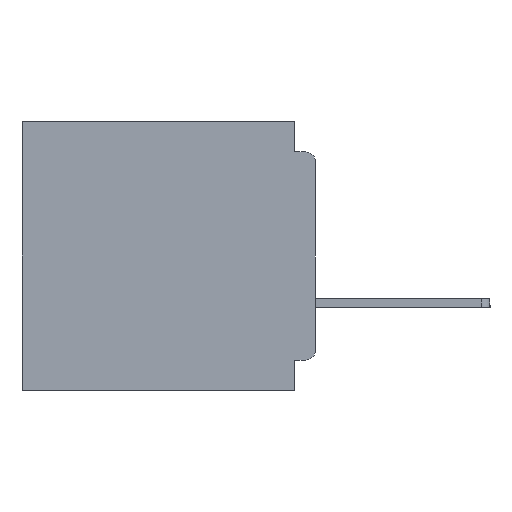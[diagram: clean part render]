
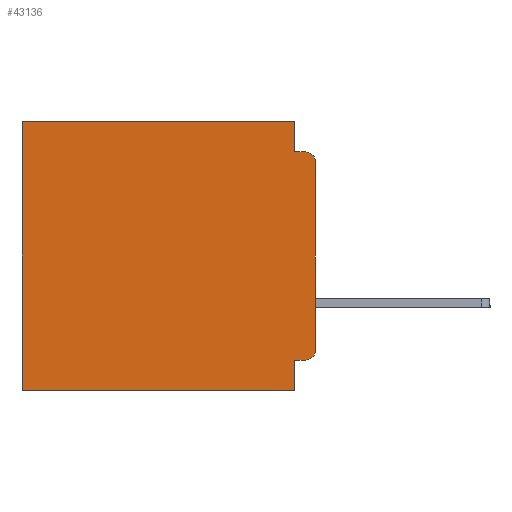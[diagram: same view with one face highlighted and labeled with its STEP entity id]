
A CAD part, left-side view. The second image highlights one B-rep face of the part: STEP entity #43136.
In plain terms, the highlighted planar face has unit normal (-1, 0, 0).
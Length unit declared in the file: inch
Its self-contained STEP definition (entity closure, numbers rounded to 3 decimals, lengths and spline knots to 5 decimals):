
#1209 = VERTEX_POINT ( 'NONE', #57532 ) ;
#2395 = DIRECTION ( 'NONE',  ( 0., 1., 0. ) ) ;
#2938 = VECTOR ( 'NONE', #21959, 39.37008 ) ;
#3122 = ORIENTED_EDGE ( 'NONE', *, *, #51574, .T. ) ;
#3294 = VECTOR ( 'NONE', #12545, 39.37008 ) ;
#3520 = DIRECTION ( 'NONE',  ( 0., 0., -1. ) ) ;
#4760 = DIRECTION ( 'NONE',  ( -1., 0., 0. ) ) ;
#5353 = ORIENTED_EDGE ( 'NONE', *, *, #50218, .F. ) ;
#6563 = CARTESIAN_POINT ( 'NONE',  ( 0.3, 0., 0. ) ) ;
#8400 = CARTESIAN_POINT ( 'NONE',  ( 0.3, 0.437, 0. ) ) ;
#9944 = VERTEX_POINT ( 'NONE', #12247 ) ;
#10645 = CARTESIAN_POINT ( 'NONE',  ( 0.3, 0., -0.4 ) ) ;
#10893 = EDGE_CURVE ( 'NONE', #55177, #16898, #20337, .T. ) ;
#11255 = ORIENTED_EDGE ( 'NONE', *, *, #14312, .F. ) ;
#11325 = DIRECTION ( 'NONE',  ( 0., 1., 0. ) ) ;
#11742 = VERTEX_POINT ( 'NONE', #34514 ) ;
#12247 = CARTESIAN_POINT ( 'NONE',  ( 0.3, 0.031, -0.4 ) ) ;
#12248 = EDGE_CURVE ( 'NONE', #55177, #11742, #18725, .T. ) ;
#12545 = DIRECTION ( 'NONE',  ( 0., 0., -1. ) ) ;
#13112 = ORIENTED_EDGE ( 'NONE', *, *, #36123, .F. ) ;
#14312 = EDGE_CURVE ( 'NONE', #32155, #57522, #51181, .T. ) ;
#15388 = EDGE_CURVE ( 'NONE', #32155, #17351, #39405, .T. ) ;
#15807 = DIRECTION ( 'NONE',  ( 0., 1., 0. ) ) ;
#16235 = ORIENTED_EDGE ( 'NONE', *, *, #10893, .T. ) ;
#16368 = CARTESIAN_POINT ( 'NONE',  ( 0.3, 0., -0.355 ) ) ;
#16898 = VERTEX_POINT ( 'NONE', #42396 ) ;
#16939 = AXIS2_PLACEMENT_3D ( 'NONE', #32776, #4760, #37482 ) ;
#17249 = LINE ( 'NONE', #49866, #3294 ) ;
#17351 = VERTEX_POINT ( 'NONE', #8400 ) ;
#17574 = DIRECTION ( 'NONE',  ( -1., 0., 0. ) ) ;
#18725 = LINE ( 'NONE', #39203, #42150 ) ;
#20140 = EDGE_CURVE ( 'NONE', #1209, #11742, #28100, .T. ) ;
#20337 = CIRCLE ( 'NONE', #16939, 0.015 ) ;
#21219 = ORIENTED_EDGE ( 'NONE', *, *, #20140, .T. ) ;
#21724 = LINE ( 'NONE', #16368, #32735 ) ;
#21959 = DIRECTION ( 'NONE',  ( 0., 0., -1. ) ) ;
#22036 = ORIENTED_EDGE ( 'NONE', *, *, #32426, .F. ) ;
#22217 = LINE ( 'NONE', #31538, #45684 ) ;
#22453 = CARTESIAN_POINT ( 'NONE',  ( 0.3, 0.031, -0.355 ) ) ;
#23153 = LINE ( 'NONE', #50986, #35647 ) ;
#23790 = CARTESIAN_POINT ( 'NONE',  ( 0.3, 0.437, -0.4 ) ) ;
#25708 = ORIENTED_EDGE ( 'NONE', *, *, #12248, .F. ) ;
#27734 = DIRECTION ( 'NONE',  ( 0., -1., 0. ) ) ;
#28100 = CIRCLE ( 'NONE', #52515, 0.015 ) ;
#29387 = DIRECTION ( 'NONE',  ( 0., 0., -1. ) ) ;
#31421 = CARTESIAN_POINT ( 'NONE',  ( 0.3, 0.031, 0. ) ) ;
#31483 = VERTEX_POINT ( 'NONE', #23790 ) ;
#31538 = CARTESIAN_POINT ( 'NONE',  ( 0.3, 0.031, -0.4 ) ) ;
#32155 = VERTEX_POINT ( 'NONE', #43239 ) ;
#32426 = EDGE_CURVE ( 'NONE', #39357, #9944, #22217, .T. ) ;
#32735 = VECTOR ( 'NONE', #2395, 39.37008 ) ;
#32776 = CARTESIAN_POINT ( 'NONE',  ( 0.3, 0.015, -0.06 ) ) ;
#33311 = LINE ( 'NONE', #48467, #56722 ) ;
#34514 = CARTESIAN_POINT ( 'NONE',  ( 0.3, 0., -0.34 ) ) ;
#34724 = AXIS2_PLACEMENT_3D ( 'NONE', #10645, #57430, #29387 ) ;
#35647 = VECTOR ( 'NONE', #27734, 39.37008 ) ;
#35848 = FACE_OUTER_BOUND ( 'NONE', #46391, .T. ) ;
#36123 = EDGE_CURVE ( 'NONE', #57522, #16898, #23153, .T. ) ;
#37439 = CARTESIAN_POINT ( 'NONE',  ( 0.3, 0.031, -0.045 ) ) ;
#37482 = DIRECTION ( 'NONE',  ( 0., 0., -1. ) ) ;
#39203 = CARTESIAN_POINT ( 'NONE',  ( 0.3, 0., -0.4 ) ) ;
#39357 = VERTEX_POINT ( 'NONE', #22453 ) ;
#39405 = LINE ( 'NONE', #6563, #51772 ) ;
#42150 = VECTOR ( 'NONE', #57998, 39.37008 ) ;
#42396 = CARTESIAN_POINT ( 'NONE',  ( 0.3, 0.015, -0.045 ) ) ;
#43136 = ADVANCED_FACE ( 'NONE', ( #35848 ), #43332, .F. ) ;
#43239 = CARTESIAN_POINT ( 'NONE',  ( 0.3, 0.031, 0. ) ) ;
#43332 = PLANE ( 'NONE',  #34724 ) ;
#45026 = ORIENTED_EDGE ( 'NONE', *, *, #15388, .T. ) ;
#45557 = CARTESIAN_POINT ( 'NONE',  ( 0.3, 0.015, -0.34 ) ) ;
#45684 = VECTOR ( 'NONE', #3520, 39.37008 ) ;
#46391 = EDGE_LOOP ( 'NONE', ( #25708, #16235, #13112, #11255, #45026, #3122, #52841, #22036, #5353, #21219 ) ) ;
#48467 = CARTESIAN_POINT ( 'NONE',  ( 0.3, 0., -0.4 ) ) ;
#49866 = CARTESIAN_POINT ( 'NONE',  ( 0.3, 0.437, -0.4 ) ) ;
#50216 = DIRECTION ( 'NONE',  ( 0., 0., -1. ) ) ;
#50218 = EDGE_CURVE ( 'NONE', #1209, #39357, #21724, .T. ) ;
#50986 = CARTESIAN_POINT ( 'NONE',  ( 0.3, 0., -0.045 ) ) ;
#51181 = LINE ( 'NONE', #31421, #2938 ) ;
#51574 = EDGE_CURVE ( 'NONE', #17351, #31483, #17249, .T. ) ;
#51772 = VECTOR ( 'NONE', #11325, 39.37008 ) ;
#52515 = AXIS2_PLACEMENT_3D ( 'NONE', #45557, #17574, #50216 ) ;
#52841 = ORIENTED_EDGE ( 'NONE', *, *, #60544, .F. ) ;
#54182 = CARTESIAN_POINT ( 'NONE',  ( 0.3, 0., -0.06 ) ) ;
#55177 = VERTEX_POINT ( 'NONE', #54182 ) ;
#56722 = VECTOR ( 'NONE', #15807, 39.37008 ) ;
#57430 = DIRECTION ( 'NONE',  ( 1., 0., 0. ) ) ;
#57522 = VERTEX_POINT ( 'NONE', #37439 ) ;
#57532 = CARTESIAN_POINT ( 'NONE',  ( 0.3, 0.015, -0.355 ) ) ;
#57998 = DIRECTION ( 'NONE',  ( 0., 0., -1. ) ) ;
#60544 = EDGE_CURVE ( 'NONE', #9944, #31483, #33311, .T. ) ;
